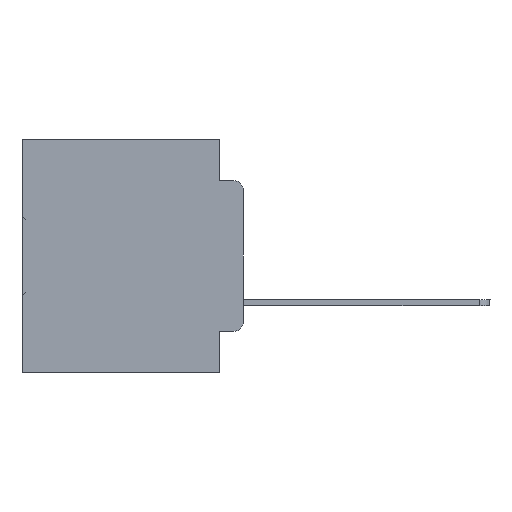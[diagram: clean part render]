
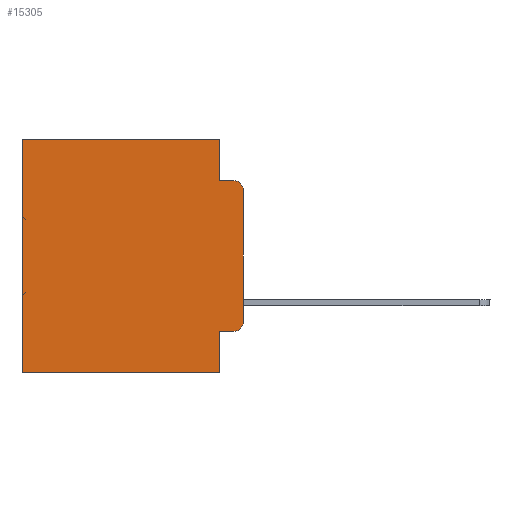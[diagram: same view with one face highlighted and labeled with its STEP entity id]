
A CAD part, left-side view. The second image highlights one B-rep face of the part: STEP entity #15305.
In plain terms, the highlighted planar face has unit normal (-1, 0, 0).
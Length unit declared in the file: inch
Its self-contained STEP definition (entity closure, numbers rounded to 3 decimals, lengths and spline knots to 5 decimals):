
#502 = VERTEX_POINT ( 'NONE', #20741 ) ;
#633 = CARTESIAN_POINT ( 'NONE',  ( 0.298, 0., -0.5 ) ) ;
#810 = LINE ( 'NONE', #8595, #13148 ) ;
#1527 = EDGE_CURVE ( 'NONE', #4168, #502, #30523, .T. ) ;
#1854 = EDGE_CURVE ( 'NONE', #34302, #30751, #16085, .T. ) ;
#1978 = CARTESIAN_POINT ( 'NONE',  ( 0.298, 0.051, -0.4115 ) ) ;
#2166 = DIRECTION ( 'NONE',  ( 0., -1., 0. ) ) ;
#2585 = AXIS2_PLACEMENT_3D ( 'NONE', #33406, #6128, #3596 ) ;
#3108 = EDGE_CURVE ( 'NONE', #4168, #19275, #11094, .T. ) ;
#3265 = PLANE ( 'NONE',  #2585 ) ;
#3596 = DIRECTION ( 'NONE',  ( 0., 0., -1. ) ) ;
#4168 = VERTEX_POINT ( 'NONE', #18519 ) ;
#4799 = EDGE_CURVE ( 'NONE', #14708, #31947, #8956, .T. ) ;
#6128 = DIRECTION ( 'NONE',  ( 1., 0., 0. ) ) ;
#6585 = DIRECTION ( 'NONE',  ( 0., 0., -1. ) ) ;
#6781 = ORIENTED_EDGE ( 'NONE', *, *, #1854, .T. ) ;
#8595 = CARTESIAN_POINT ( 'NONE',  ( 0.298, 0.473, 0. ) ) ;
#8640 = VERTEX_POINT ( 'NONE', #22137 ) ;
#8956 = LINE ( 'NONE', #11662, #10605 ) ;
#9797 = ORIENTED_EDGE ( 'NONE', *, *, #21358, .F. ) ;
#10100 = VECTOR ( 'NONE', #13981, 39.37008 ) ;
#10554 = CARTESIAN_POINT ( 'NONE',  ( 0.298, 0.473, 0. ) ) ;
#10605 = VECTOR ( 'NONE', #6585, 39.37008 ) ;
#11066 = DIRECTION ( 'NONE',  ( -1., 0., 0. ) ) ;
#11094 = LINE ( 'NONE', #16868, #10100 ) ;
#11662 = CARTESIAN_POINT ( 'NONE',  ( 0.298, 0.051, 0. ) ) ;
#11691 = EDGE_CURVE ( 'NONE', #34302, #15344, #15532, .T. ) ;
#12464 = EDGE_CURVE ( 'NONE', #15344, #502, #30299, .T. ) ;
#13148 = VECTOR ( 'NONE', #30621, 39.37008 ) ;
#13981 = DIRECTION ( 'NONE',  ( 0., 0., -1. ) ) ;
#14708 = VERTEX_POINT ( 'NONE', #32226 ) ;
#14946 = AXIS2_PLACEMENT_3D ( 'NONE', #21913, #11066, #32915 ) ;
#15305 = ADVANCED_FACE ( 'NONE', ( #28340 ), #3265, .F. ) ;
#15344 = VERTEX_POINT ( 'NONE', #22924 ) ;
#15532 = LINE ( 'NONE', #23666, #32911 ) ;
#16085 = LINE ( 'NONE', #32167, #29446 ) ;
#16638 = CARTESIAN_POINT ( 'NONE',  ( 0.298, 0.02, -0.4115 ) ) ;
#16868 = CARTESIAN_POINT ( 'NONE',  ( 0.298, 0., 0. ) ) ;
#17060 = ORIENTED_EDGE ( 'NONE', *, *, #32732, .T. ) ;
#18245 = VERTEX_POINT ( 'NONE', #16638 ) ;
#18519 = CARTESIAN_POINT ( 'NONE',  ( 0.298, 0., -0.1085 ) ) ;
#18622 = EDGE_LOOP ( 'NONE', ( #32557, #23296, #25332, #21841, #6781, #34011, #9797, #21703, #23328, #17060 ) ) ;
#18675 = EDGE_CURVE ( 'NONE', #30751, #8640, #810, .T. ) ;
#19275 = VERTEX_POINT ( 'NONE', #28892 ) ;
#19906 = DIRECTION ( 'NONE',  ( -1., 0., 0. ) ) ;
#20741 = CARTESIAN_POINT ( 'NONE',  ( 0.298, 0.02, -0.0885 ) ) ;
#20799 = DIRECTION ( 'NONE',  ( 0., 1., 0. ) ) ;
#20973 = DIRECTION ( 'NONE',  ( 0., 0., -1. ) ) ;
#21358 = EDGE_CURVE ( 'NONE', #31947, #8640, #22866, .T. ) ;
#21385 = CARTESIAN_POINT ( 'NONE',  ( 0.298, 0.051, 0. ) ) ;
#21703 = ORIENTED_EDGE ( 'NONE', *, *, #4799, .F. ) ;
#21841 = ORIENTED_EDGE ( 'NONE', *, *, #11691, .F. ) ;
#21913 = CARTESIAN_POINT ( 'NONE',  ( 0.298, 0.02, -0.1085 ) ) ;
#22137 = CARTESIAN_POINT ( 'NONE',  ( 0.298, 0.473, -0.5 ) ) ;
#22604 = VECTOR ( 'NONE', #25240, 39.37008 ) ;
#22617 = CARTESIAN_POINT ( 'NONE',  ( 0.298, 0.02, -0.3915 ) ) ;
#22704 = CIRCLE ( 'NONE', #31321, 0.02 ) ;
#22866 = LINE ( 'NONE', #633, #29472 ) ;
#22924 = CARTESIAN_POINT ( 'NONE',  ( 0.298, 0.051, -0.0885 ) ) ;
#23296 = ORIENTED_EDGE ( 'NONE', *, *, #1527, .T. ) ;
#23328 = ORIENTED_EDGE ( 'NONE', *, *, #27066, .T. ) ;
#23356 = VECTOR ( 'NONE', #2166, 39.37008 ) ;
#23666 = CARTESIAN_POINT ( 'NONE',  ( 0.298, 0.051, 0. ) ) ;
#25240 = DIRECTION ( 'NONE',  ( 0., -1., 0. ) ) ;
#25332 = ORIENTED_EDGE ( 'NONE', *, *, #12464, .F. ) ;
#26746 = CARTESIAN_POINT ( 'NONE',  ( 0.298, 0.051, -0.5 ) ) ;
#26907 = LINE ( 'NONE', #1978, #23356 ) ;
#27066 = EDGE_CURVE ( 'NONE', #14708, #18245, #26907, .T. ) ;
#28340 = FACE_OUTER_BOUND ( 'NONE', #18622, .T. ) ;
#28892 = CARTESIAN_POINT ( 'NONE',  ( 0.298, 0., -0.3915 ) ) ;
#29446 = VECTOR ( 'NONE', #20799, 39.37008 ) ;
#29472 = VECTOR ( 'NONE', #33863, 39.37008 ) ;
#30299 = LINE ( 'NONE', #33351, #22604 ) ;
#30523 = CIRCLE ( 'NONE', #14946, 0.02 ) ;
#30621 = DIRECTION ( 'NONE',  ( 0., 0., -1. ) ) ;
#30751 = VERTEX_POINT ( 'NONE', #10554 ) ;
#30914 = DIRECTION ( 'NONE',  ( 0., 0., -1. ) ) ;
#31321 = AXIS2_PLACEMENT_3D ( 'NONE', #22617, #19906, #30914 ) ;
#31947 = VERTEX_POINT ( 'NONE', #26746 ) ;
#32167 = CARTESIAN_POINT ( 'NONE',  ( 0.298, 0., 0. ) ) ;
#32226 = CARTESIAN_POINT ( 'NONE',  ( 0.298, 0.051, -0.4115 ) ) ;
#32557 = ORIENTED_EDGE ( 'NONE', *, *, #3108, .F. ) ;
#32732 = EDGE_CURVE ( 'NONE', #18245, #19275, #22704, .T. ) ;
#32911 = VECTOR ( 'NONE', #20973, 39.37008 ) ;
#32915 = DIRECTION ( 'NONE',  ( 0., 0., -1. ) ) ;
#33351 = CARTESIAN_POINT ( 'NONE',  ( 0.298, 0.051, -0.0885 ) ) ;
#33406 = CARTESIAN_POINT ( 'NONE',  ( 0.298, 0., 0. ) ) ;
#33863 = DIRECTION ( 'NONE',  ( 0., 1., 0. ) ) ;
#34011 = ORIENTED_EDGE ( 'NONE', *, *, #18675, .T. ) ;
#34302 = VERTEX_POINT ( 'NONE', #21385 ) ;
